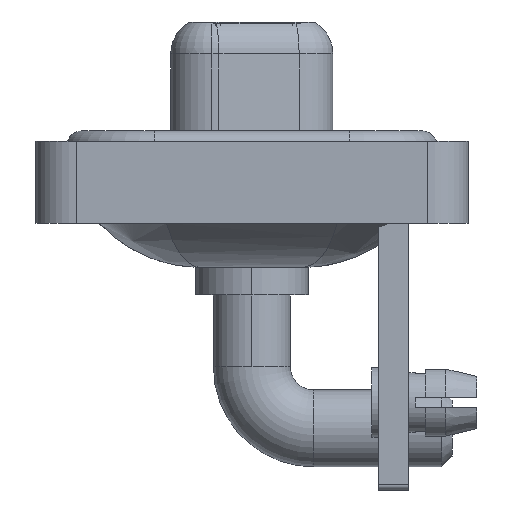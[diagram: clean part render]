
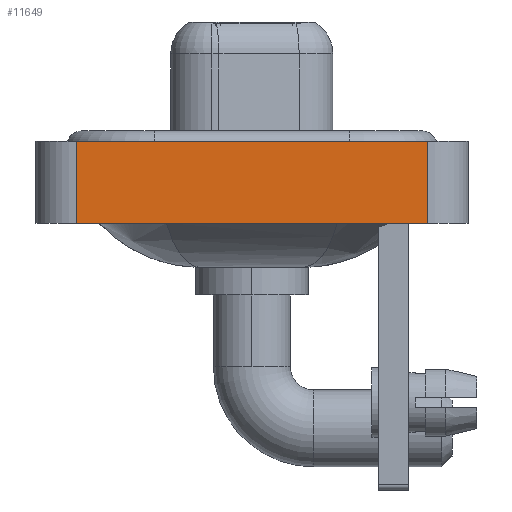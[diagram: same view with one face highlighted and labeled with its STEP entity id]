
A CAD part, left-side view. The second image highlights one B-rep face of the part: STEP entity #11649.
In plain terms, the highlighted planar face has unit normal (-1, 0, 0).
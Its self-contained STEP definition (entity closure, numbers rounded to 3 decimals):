
#338 = ORIENTED_EDGE ( 'NONE', *, *, #8975, .T. ) ;
#396 = CARTESIAN_POINT ( 'NONE',  ( -7.3, -8.55, -3.6 ) ) ;
#468 = ORIENTED_EDGE ( 'NONE', *, *, #11150, .F. ) ;
#2112 = CARTESIAN_POINT ( 'NONE',  ( -7.3, 8.55, -3.6 ) ) ;
#2978 = AXIS2_PLACEMENT_3D ( 'NONE', #396, #13167, #17663 ) ;
#3320 = DIRECTION ( 'NONE',  ( 0., 0., 1. ) ) ;
#3417 = CARTESIAN_POINT ( 'NONE',  ( -7.3, -8.55, -3.6 ) ) ;
#5419 = DIRECTION ( 'NONE',  ( 0., -1., 0. ) ) ;
#7415 = VERTEX_POINT ( 'NONE', #17966 ) ;
#8874 = FACE_OUTER_BOUND ( 'NONE', #17684, .T. ) ;
#8907 = VECTOR ( 'NONE', #3320, 1000. ) ;
#8975 = EDGE_CURVE ( 'NONE', #7415, #12404, #17609, .T. ) ;
#9086 = DIRECTION ( 'NONE',  ( 0., 0., 1. ) ) ;
#9099 = EDGE_CURVE ( 'NONE', #9481, #12404, #16570, .T. ) ;
#9451 = DIRECTION ( 'NONE',  ( 0., -1., 0. ) ) ;
#9481 = VERTEX_POINT ( 'NONE', #15226 ) ;
#9756 = CARTESIAN_POINT ( 'NONE',  ( -7.3, -8.55, 0.4 ) ) ;
#10312 = VECTOR ( 'NONE', #5419, 1000. ) ;
#10800 = CARTESIAN_POINT ( 'NONE',  ( -7.3, 8.55, -3.6 ) ) ;
#11150 = EDGE_CURVE ( 'NONE', #15980, #9481, #11977, .T. ) ;
#11649 = ADVANCED_FACE ( 'NONE', ( #8874 ), #17302, .T. ) ;
#11937 = ORIENTED_EDGE ( 'NONE', *, *, #9099, .F. ) ;
#11977 = LINE ( 'NONE', #2112, #8907 ) ;
#12404 = VERTEX_POINT ( 'NONE', #9756 ) ;
#12491 = LINE ( 'NONE', #15301, #10312 ) ;
#13167 = DIRECTION ( 'NONE',  ( -1., 0., 0. ) ) ;
#13663 = CARTESIAN_POINT ( 'NONE',  ( -7.3, -8.55, 0.4 ) ) ;
#15226 = CARTESIAN_POINT ( 'NONE',  ( -7.3, 8.55, 0.4 ) ) ;
#15301 = CARTESIAN_POINT ( 'NONE',  ( -7.3, -8.55, -3.6 ) ) ;
#15359 = VECTOR ( 'NONE', #9086, 1000. ) ;
#15631 = EDGE_CURVE ( 'NONE', #15980, #7415, #12491, .T. ) ;
#15879 = ORIENTED_EDGE ( 'NONE', *, *, #15631, .T. ) ;
#15960 = VECTOR ( 'NONE', #9451, 1000. ) ;
#15980 = VERTEX_POINT ( 'NONE', #10800 ) ;
#16570 = LINE ( 'NONE', #13663, #15960 ) ;
#17302 = PLANE ( 'NONE',  #2978 ) ;
#17609 = LINE ( 'NONE', #3417, #15359 ) ;
#17663 = DIRECTION ( 'NONE',  ( 0., 0., 1. ) ) ;
#17684 = EDGE_LOOP ( 'NONE', ( #338, #11937, #468, #15879 ) ) ;
#17966 = CARTESIAN_POINT ( 'NONE',  ( -7.3, -8.55, -3.6 ) ) ;
